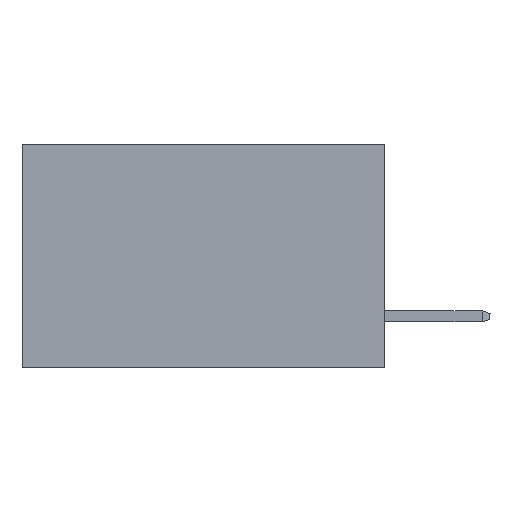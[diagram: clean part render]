
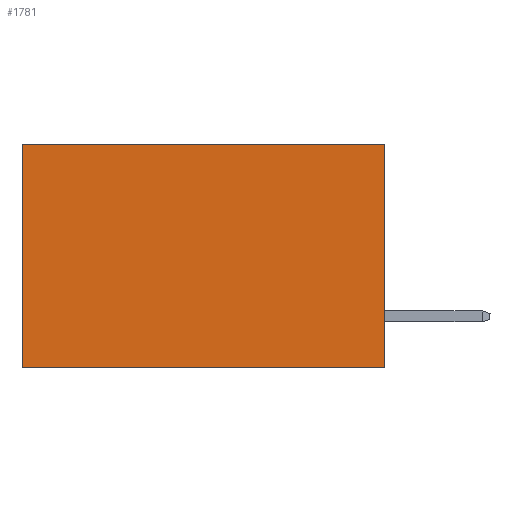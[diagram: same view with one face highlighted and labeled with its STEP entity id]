
A CAD part, left-side view. The second image highlights one B-rep face of the part: STEP entity #1781.
In plain terms, the highlighted planar face has unit normal (-1, 0, 0).
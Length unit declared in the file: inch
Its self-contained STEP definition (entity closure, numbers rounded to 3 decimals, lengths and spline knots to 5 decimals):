
#389 = AXIS2_PLACEMENT_3D ( 'NONE', #7628, #7698, #1370 ) ;
#467 = LINE ( 'NONE', #7762, #964 ) ;
#715 = CARTESIAN_POINT ( 'NONE',  ( 0.298, 0., -0.37 ) ) ;
#872 = CARTESIAN_POINT ( 'NONE',  ( 0.298, 0.6, 0. ) ) ;
#964 = VECTOR ( 'NONE', #6270, 39.37008 ) ;
#1092 = CARTESIAN_POINT ( 'NONE',  ( 0.298, 0., 0. ) ) ;
#1111 = VERTEX_POINT ( 'NONE', #872 ) ;
#1245 = ORIENTED_EDGE ( 'NONE', *, *, #3424, .T. ) ;
#1370 = DIRECTION ( 'NONE',  ( 0., 0., -1. ) ) ;
#1781 = ADVANCED_FACE ( 'NONE', ( #8243 ), #6132, .F. ) ;
#1879 = DIRECTION ( 'NONE',  ( 0., 1., 0. ) ) ;
#2221 = LINE ( 'NONE', #1092, #9983 ) ;
#2514 = LINE ( 'NONE', #4668, #4875 ) ;
#3424 = EDGE_CURVE ( 'NONE', #1111, #6419, #2514, .T. ) ;
#3447 = EDGE_CURVE ( 'NONE', #8308, #7727, #467, .T. ) ;
#3906 = CARTESIAN_POINT ( 'NONE',  ( 0.298, 0., 0. ) ) ;
#4046 = CARTESIAN_POINT ( 'NONE',  ( 0.298, 0., -0.37 ) ) ;
#4639 = DIRECTION ( 'NONE',  ( 0., 0., -1. ) ) ;
#4668 = CARTESIAN_POINT ( 'NONE',  ( 0.298, 0.6, 0. ) ) ;
#4875 = VECTOR ( 'NONE', #4639, 39.37008 ) ;
#5139 = EDGE_CURVE ( 'NONE', #8308, #1111, #2221, .T. ) ;
#5542 = ORIENTED_EDGE ( 'NONE', *, *, #5139, .T. ) ;
#5554 = ORIENTED_EDGE ( 'NONE', *, *, #3447, .F. ) ;
#5555 = VECTOR ( 'NONE', #8644, 39.37008 ) ;
#6108 = EDGE_CURVE ( 'NONE', #7727, #6419, #6432, .T. ) ;
#6132 = PLANE ( 'NONE',  #389 ) ;
#6270 = DIRECTION ( 'NONE',  ( 0., 0., -1. ) ) ;
#6419 = VERTEX_POINT ( 'NONE', #8208 ) ;
#6432 = LINE ( 'NONE', #4046, #5555 ) ;
#6820 = ORIENTED_EDGE ( 'NONE', *, *, #6108, .F. ) ;
#7628 = CARTESIAN_POINT ( 'NONE',  ( 0.298, 0., 0. ) ) ;
#7698 = DIRECTION ( 'NONE',  ( 1., 0., 0. ) ) ;
#7727 = VERTEX_POINT ( 'NONE', #715 ) ;
#7762 = CARTESIAN_POINT ( 'NONE',  ( 0.298, 0., 0. ) ) ;
#8208 = CARTESIAN_POINT ( 'NONE',  ( 0.298, 0.6, -0.37 ) ) ;
#8243 = FACE_OUTER_BOUND ( 'NONE', #9004, .T. ) ;
#8308 = VERTEX_POINT ( 'NONE', #3906 ) ;
#8644 = DIRECTION ( 'NONE',  ( 0., 1., 0. ) ) ;
#9004 = EDGE_LOOP ( 'NONE', ( #1245, #6820, #5554, #5542 ) ) ;
#9983 = VECTOR ( 'NONE', #1879, 39.37008 ) ;
